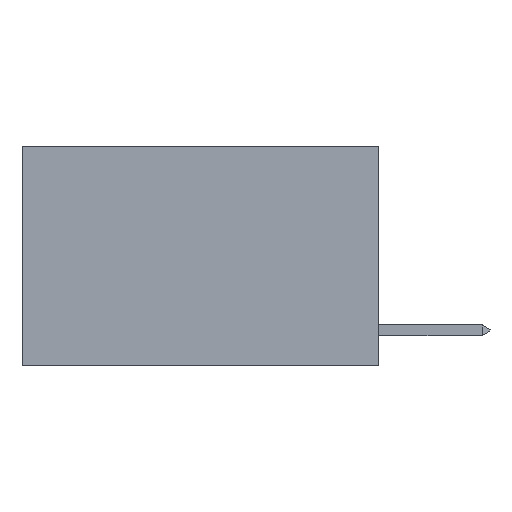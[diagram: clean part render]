
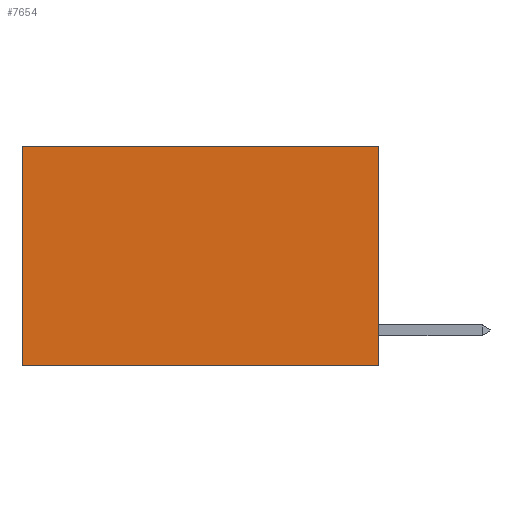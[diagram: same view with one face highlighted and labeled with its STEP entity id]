
A CAD part, left-side view. The second image highlights one B-rep face of the part: STEP entity #7654.
In plain terms, the highlighted planar face has unit normal (-1, 0, 0).
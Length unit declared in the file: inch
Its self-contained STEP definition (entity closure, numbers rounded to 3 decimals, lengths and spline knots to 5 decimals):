
#1085 = VERTEX_POINT ( 'NONE', #8293 ) ;
#1728 = VECTOR ( 'NONE', #8393, 39.37008 ) ;
#2152 = LINE ( 'NONE', #12847, #14662 ) ;
#2430 = CARTESIAN_POINT ( 'NONE',  ( 0.2625, 0., -0.37 ) ) ;
#2611 = VERTEX_POINT ( 'NONE', #13823 ) ;
#3562 = EDGE_CURVE ( 'NONE', #5492, #7496, #8182, .T. ) ;
#3616 = DIRECTION ( 'NONE',  ( 0., 0., -1. ) ) ;
#4350 = DIRECTION ( 'NONE',  ( 0., 0., -1. ) ) ;
#4511 = CARTESIAN_POINT ( 'NONE',  ( 0.2625, 0.6, 0. ) ) ;
#4919 = VECTOR ( 'NONE', #13322, 39.37008 ) ;
#5487 = EDGE_CURVE ( 'NONE', #7496, #2611, #2152, .T. ) ;
#5492 = VERTEX_POINT ( 'NONE', #9252 ) ;
#6336 = VECTOR ( 'NONE', #11859, 39.37008 ) ;
#7144 = CARTESIAN_POINT ( 'NONE',  ( 0.2625, 0., 0. ) ) ;
#7496 = VERTEX_POINT ( 'NONE', #4511 ) ;
#7654 = ADVANCED_FACE ( 'NONE', ( #14592 ), #8447, .F. ) ;
#7681 = EDGE_CURVE ( 'NONE', #1085, #2611, #11777, .T. ) ;
#8182 = LINE ( 'NONE', #7144, #1728 ) ;
#8293 = CARTESIAN_POINT ( 'NONE',  ( 0.2625, 0., -0.37 ) ) ;
#8393 = DIRECTION ( 'NONE',  ( 0., 1., 0. ) ) ;
#8447 = PLANE ( 'NONE',  #12273 ) ;
#9218 = LINE ( 'NONE', #11802, #6336 ) ;
#9252 = CARTESIAN_POINT ( 'NONE',  ( 0.2625, 0., 0. ) ) ;
#9664 = CARTESIAN_POINT ( 'NONE',  ( 0.2625, 0., 0. ) ) ;
#10906 = DIRECTION ( 'NONE',  ( 1., 0., 0. ) ) ;
#11777 = LINE ( 'NONE', #2430, #4919 ) ;
#11802 = CARTESIAN_POINT ( 'NONE',  ( 0.2625, 0., 0. ) ) ;
#11859 = DIRECTION ( 'NONE',  ( 0., 0., -1. ) ) ;
#12273 = AXIS2_PLACEMENT_3D ( 'NONE', #9664, #10906, #3616 ) ;
#12368 = ORIENTED_EDGE ( 'NONE', *, *, #3562, .T. ) ;
#12487 = ORIENTED_EDGE ( 'NONE', *, *, #13632, .F. ) ;
#12847 = CARTESIAN_POINT ( 'NONE',  ( 0.2625, 0.6, 0. ) ) ;
#13322 = DIRECTION ( 'NONE',  ( 0., 1., 0. ) ) ;
#13632 = EDGE_CURVE ( 'NONE', #5492, #1085, #9218, .T. ) ;
#13823 = CARTESIAN_POINT ( 'NONE',  ( 0.2625, 0.6, -0.37 ) ) ;
#14019 = ORIENTED_EDGE ( 'NONE', *, *, #5487, .T. ) ;
#14141 = ORIENTED_EDGE ( 'NONE', *, *, #7681, .F. ) ;
#14287 = EDGE_LOOP ( 'NONE', ( #14019, #14141, #12487, #12368 ) ) ;
#14592 = FACE_OUTER_BOUND ( 'NONE', #14287, .T. ) ;
#14662 = VECTOR ( 'NONE', #4350, 39.37008 ) ;
